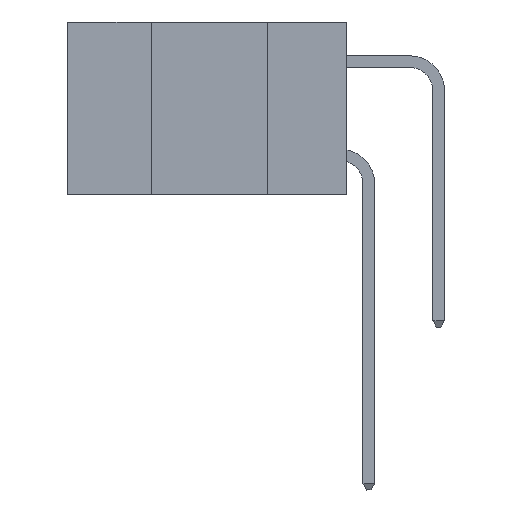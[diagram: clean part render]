
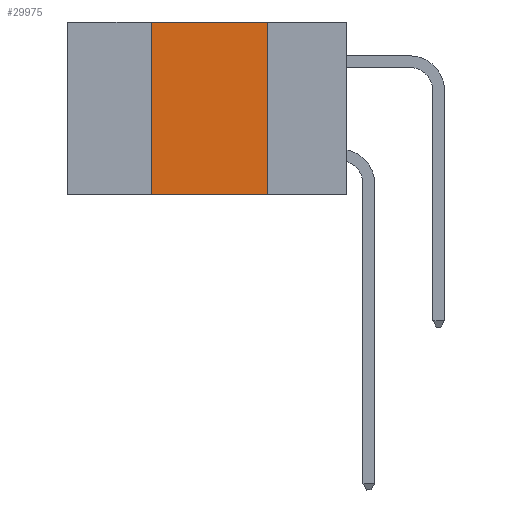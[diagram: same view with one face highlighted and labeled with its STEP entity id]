
A CAD part, left-side view. The second image highlights one B-rep face of the part: STEP entity #29975.
In plain terms, the highlighted planar face has unit normal (-1, 0, 0).
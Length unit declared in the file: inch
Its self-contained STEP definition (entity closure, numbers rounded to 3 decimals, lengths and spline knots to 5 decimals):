
#771 = CARTESIAN_POINT ( 'NONE',  ( 0., 0.42, 0. ) ) ;
#2761 = DIRECTION ( 'NONE',  ( 1., 0., 0. ) ) ;
#3294 = DIRECTION ( 'NONE',  ( 0., 0., -1. ) ) ;
#3750 = VECTOR ( 'NONE', #8623, 39.37008 ) ;
#3871 = ORIENTED_EDGE ( 'NONE', *, *, #25594, .F. ) ;
#4102 = EDGE_CURVE ( 'NONE', #18172, #12792, #16272, .T. ) ;
#4233 = ORIENTED_EDGE ( 'NONE', *, *, #18524, .F. ) ;
#6860 = LINE ( 'NONE', #15025, #27396 ) ;
#8623 = DIRECTION ( 'NONE',  ( 0., 0., 1. ) ) ;
#9576 = CARTESIAN_POINT ( 'NONE',  ( 0., 0.17, -0.37 ) ) ;
#10947 = PLANE ( 'NONE',  #29293 ) ;
#12408 = EDGE_CURVE ( 'NONE', #18172, #26799, #6860, .T. ) ;
#12792 = VERTEX_POINT ( 'NONE', #771 ) ;
#14275 = LINE ( 'NONE', #28012, #27807 ) ;
#15025 = CARTESIAN_POINT ( 'NONE',  ( 0., 0.6, -0.37 ) ) ;
#16272 = LINE ( 'NONE', #19315, #3750 ) ;
#18172 = VERTEX_POINT ( 'NONE', #30869 ) ;
#18320 = ORIENTED_EDGE ( 'NONE', *, *, #4102, .F. ) ;
#18524 = EDGE_CURVE ( 'NONE', #12792, #28339, #26742, .T. ) ;
#18886 = DIRECTION ( 'NONE',  ( 0., -1., 0. ) ) ;
#19315 = CARTESIAN_POINT ( 'NONE',  ( 0., 0.42, 0. ) ) ;
#20044 = DIRECTION ( 'NONE',  ( 0., -1., 0. ) ) ;
#22396 = VECTOR ( 'NONE', #18886, 39.37008 ) ;
#24990 = DIRECTION ( 'NONE',  ( 0., 0., -1. ) ) ;
#25594 = EDGE_CURVE ( 'NONE', #28339, #26799, #14275, .T. ) ;
#26742 = LINE ( 'NONE', #30302, #22396 ) ;
#26799 = VERTEX_POINT ( 'NONE', #9576 ) ;
#27396 = VECTOR ( 'NONE', #20044, 39.37008 ) ;
#27807 = VECTOR ( 'NONE', #24990, 39.37008 ) ;
#27879 = FACE_OUTER_BOUND ( 'NONE', #32022, .T. ) ;
#28012 = CARTESIAN_POINT ( 'NONE',  ( 0., 0.17, 0. ) ) ;
#28339 = VERTEX_POINT ( 'NONE', #33441 ) ;
#29293 = AXIS2_PLACEMENT_3D ( 'NONE', #30549, #2761, #3294 ) ;
#29975 = ADVANCED_FACE ( 'NONE', ( #27879 ), #10947, .F. ) ;
#30302 = CARTESIAN_POINT ( 'NONE',  ( 0., 0.6, 0. ) ) ;
#30549 = CARTESIAN_POINT ( 'NONE',  ( 0., 0.6, 0. ) ) ;
#30869 = CARTESIAN_POINT ( 'NONE',  ( 0., 0.42, -0.37 ) ) ;
#32022 = EDGE_LOOP ( 'NONE', ( #3871, #4233, #18320, #32415 ) ) ;
#32415 = ORIENTED_EDGE ( 'NONE', *, *, #12408, .T. ) ;
#33441 = CARTESIAN_POINT ( 'NONE',  ( 0., 0.17, 0. ) ) ;
